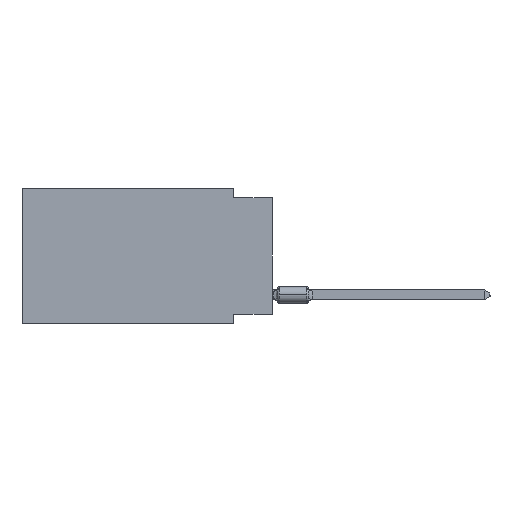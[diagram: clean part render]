
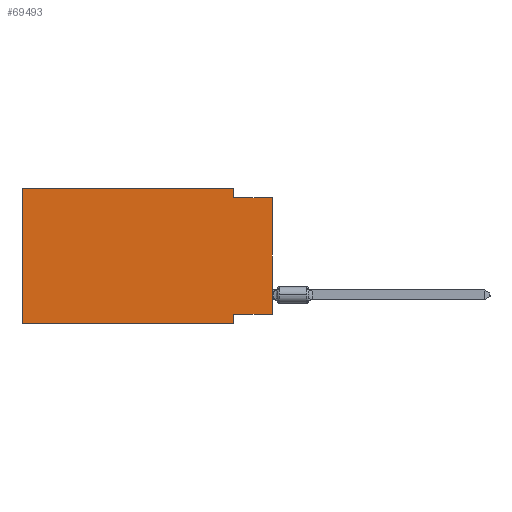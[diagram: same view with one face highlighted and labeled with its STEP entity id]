
A CAD part, left-side view. The second image highlights one B-rep face of the part: STEP entity #69493.
In plain terms, the highlighted planar face has unit normal (-1, 0, 0).
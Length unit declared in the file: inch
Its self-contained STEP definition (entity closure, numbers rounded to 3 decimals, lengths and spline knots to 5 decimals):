
#704 = VECTOR ( 'NONE', #65677, 39.37008 ) ;
#1087 = DIRECTION ( 'NONE',  ( 0., 0., -1. ) ) ;
#1253 = ORIENTED_EDGE ( 'NONE', *, *, #34257, .F. ) ;
#1753 = CARTESIAN_POINT ( 'NONE',  ( 0., 0., 0. ) ) ;
#1816 = DIRECTION ( 'NONE',  ( 1., 0., 0. ) ) ;
#3153 = ORIENTED_EDGE ( 'NONE', *, *, #6699, .F. ) ;
#4096 = AXIS2_PLACEMENT_3D ( 'NONE', #7172, #1816, #1087 ) ;
#5182 = ORIENTED_EDGE ( 'NONE', *, *, #66486, .F. ) ;
#6467 = PLANE ( 'NONE',  #4096 ) ;
#6699 = EDGE_CURVE ( 'NONE', #68010, #12675, #28112, .T. ) ;
#6982 = EDGE_CURVE ( 'NONE', #12675, #67169, #63118, .T. ) ;
#7172 = CARTESIAN_POINT ( 'NONE',  ( 0., 0.645, 0. ) ) ;
#10199 = VERTEX_POINT ( 'NONE', #33479 ) ;
#10296 = VECTOR ( 'NONE', #62104, 39.37008 ) ;
#12090 = EDGE_CURVE ( 'NONE', #64496, #65059, #49834, .T. ) ;
#12675 = VERTEX_POINT ( 'NONE', #52825 ) ;
#14125 = CARTESIAN_POINT ( 'NONE',  ( 0., 0.1, 0. ) ) ;
#14715 = ORIENTED_EDGE ( 'NONE', *, *, #49660, .F. ) ;
#15243 = ORIENTED_EDGE ( 'NONE', *, *, #45149, .T. ) ;
#15438 = DIRECTION ( 'NONE',  ( 0., 0., 1. ) ) ;
#15601 = EDGE_LOOP ( 'NONE', ( #15243, #1253, #29787, #3153, #14715, #55537, #5182, #54722 ) ) ;
#17204 = CARTESIAN_POINT ( 'NONE',  ( 0., 0.645, -0.35 ) ) ;
#22035 = CARTESIAN_POINT ( 'NONE',  ( 0., 0.645, 0. ) ) ;
#23984 = LINE ( 'NONE', #17204, #64839 ) ;
#24872 = LINE ( 'NONE', #46667, #43901 ) ;
#28112 = LINE ( 'NONE', #22035, #704 ) ;
#29166 = CARTESIAN_POINT ( 'NONE',  ( 0., 0.1, -0.325 ) ) ;
#29787 = ORIENTED_EDGE ( 'NONE', *, *, #6982, .F. ) ;
#33479 = CARTESIAN_POINT ( 'NONE',  ( 0., 0.1, -0.35 ) ) ;
#34257 = EDGE_CURVE ( 'NONE', #67169, #56697, #57092, .T. ) ;
#34318 = FACE_OUTER_BOUND ( 'NONE', #15601, .T. ) ;
#34570 = CARTESIAN_POINT ( 'NONE',  ( 0., 0.1, -0.025 ) ) ;
#35911 = DIRECTION ( 'NONE',  ( 0., 0., -1. ) ) ;
#36370 = VECTOR ( 'NONE', #56459, 39.37008 ) ;
#40629 = CARTESIAN_POINT ( 'NONE',  ( 0., 0., -0.025 ) ) ;
#40734 = CARTESIAN_POINT ( 'NONE',  ( 0., 0., -0.025 ) ) ;
#40742 = CARTESIAN_POINT ( 'NONE',  ( 0., 0.645, 0. ) ) ;
#40862 = EDGE_CURVE ( 'NONE', #53435, #10199, #23984, .T. ) ;
#43901 = VECTOR ( 'NONE', #35911, 39.37008 ) ;
#45149 = EDGE_CURVE ( 'NONE', #64496, #56697, #45712, .T. ) ;
#45712 = LINE ( 'NONE', #1753, #36370 ) ;
#45796 = DIRECTION ( 'NONE',  ( 0., -1., 0. ) ) ;
#46667 = CARTESIAN_POINT ( 'NONE',  ( 0., 0.1, -0.35 ) ) ;
#49660 = EDGE_CURVE ( 'NONE', #53435, #68010, #57394, .T. ) ;
#49834 = LINE ( 'NONE', #60220, #53190 ) ;
#52825 = CARTESIAN_POINT ( 'NONE',  ( 0., 0.1, 0. ) ) ;
#53190 = VECTOR ( 'NONE', #66280, 39.37008 ) ;
#53435 = VERTEX_POINT ( 'NONE', #54483 ) ;
#54483 = CARTESIAN_POINT ( 'NONE',  ( 0., 0.645, -0.35 ) ) ;
#54486 = CARTESIAN_POINT ( 'NONE',  ( 0., 0., -0.325 ) ) ;
#54722 = ORIENTED_EDGE ( 'NONE', *, *, #12090, .F. ) ;
#55537 = ORIENTED_EDGE ( 'NONE', *, *, #40862, .T. ) ;
#56459 = DIRECTION ( 'NONE',  ( 0., 0., 1. ) ) ;
#56697 = VERTEX_POINT ( 'NONE', #40734 ) ;
#57092 = LINE ( 'NONE', #40629, #10296 ) ;
#57394 = LINE ( 'NONE', #68152, #61968 ) ;
#60220 = CARTESIAN_POINT ( 'NONE',  ( 0., 0., -0.325 ) ) ;
#61968 = VECTOR ( 'NONE', #15438, 39.37008 ) ;
#62104 = DIRECTION ( 'NONE',  ( 0., -1., 0. ) ) ;
#63118 = LINE ( 'NONE', #14125, #70439 ) ;
#64496 = VERTEX_POINT ( 'NONE', #54486 ) ;
#64839 = VECTOR ( 'NONE', #45796, 39.37008 ) ;
#65059 = VERTEX_POINT ( 'NONE', #29166 ) ;
#65677 = DIRECTION ( 'NONE',  ( 0., -1., 0. ) ) ;
#66280 = DIRECTION ( 'NONE',  ( 0., 1., 0. ) ) ;
#66486 = EDGE_CURVE ( 'NONE', #65059, #10199, #24872, .T. ) ;
#67169 = VERTEX_POINT ( 'NONE', #34570 ) ;
#68010 = VERTEX_POINT ( 'NONE', #40742 ) ;
#68152 = CARTESIAN_POINT ( 'NONE',  ( 0., 0.645, 0. ) ) ;
#69493 = ADVANCED_FACE ( 'NONE', ( #34318 ), #6467, .F. ) ;
#69537 = DIRECTION ( 'NONE',  ( 0., 0., -1. ) ) ;
#70439 = VECTOR ( 'NONE', #69537, 39.37008 ) ;
